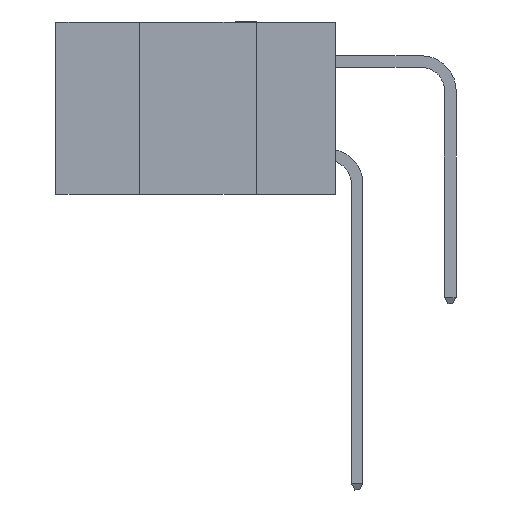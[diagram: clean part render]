
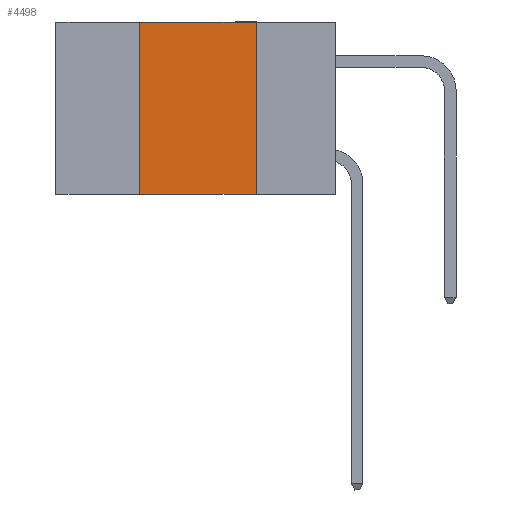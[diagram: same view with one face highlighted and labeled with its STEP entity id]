
A CAD part, left-side view. The second image highlights one B-rep face of the part: STEP entity #4498.
In plain terms, the highlighted planar face has unit normal (-1, 0, 0).
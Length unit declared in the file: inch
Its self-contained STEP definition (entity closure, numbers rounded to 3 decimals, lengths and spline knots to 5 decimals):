
#15 = VECTOR ( 'NONE', #17044, 39.37008 ) ;
#865 = FACE_OUTER_BOUND ( 'NONE', #1380, .T. ) ;
#1380 = EDGE_LOOP ( 'NONE', ( #13947, #5022, #17632, #9290 ) ) ;
#1497 = VECTOR ( 'NONE', #4788, 39.37008 ) ;
#2486 = CARTESIAN_POINT ( 'NONE',  ( 0., 0.42, -0.37 ) ) ;
#2510 = CARTESIAN_POINT ( 'NONE',  ( 0., 0.42, 0. ) ) ;
#3228 = CARTESIAN_POINT ( 'NONE',  ( 0., 0.6, -0.37 ) ) ;
#3567 = EDGE_CURVE ( 'NONE', #5511, #6806, #6130, .T. ) ;
#4498 = ADVANCED_FACE ( 'NONE', ( #865 ), #13098, .F. ) ;
#4788 = DIRECTION ( 'NONE',  ( 0., -1., 0. ) ) ;
#5022 = ORIENTED_EDGE ( 'NONE', *, *, #3567, .F. ) ;
#5511 = VERTEX_POINT ( 'NONE', #2510 ) ;
#6021 = CARTESIAN_POINT ( 'NONE',  ( 0., 0.6, 0. ) ) ;
#6130 = LINE ( 'NONE', #6021, #9954 ) ;
#6806 = VERTEX_POINT ( 'NONE', #15400 ) ;
#8310 = EDGE_CURVE ( 'NONE', #6806, #14572, #15387, .T. ) ;
#8398 = LINE ( 'NONE', #16197, #11627 ) ;
#8873 = AXIS2_PLACEMENT_3D ( 'NONE', #12870, #13113, #12237 ) ;
#9290 = ORIENTED_EDGE ( 'NONE', *, *, #15578, .T. ) ;
#9471 = LINE ( 'NONE', #3228, #1497 ) ;
#9954 = VECTOR ( 'NONE', #17787, 39.37008 ) ;
#11627 = VECTOR ( 'NONE', #12243, 39.37008 ) ;
#12237 = DIRECTION ( 'NONE',  ( 0., 0., -1. ) ) ;
#12243 = DIRECTION ( 'NONE',  ( 0., 0., 1. ) ) ;
#12870 = CARTESIAN_POINT ( 'NONE',  ( 0., 0.6, 0. ) ) ;
#12961 = CARTESIAN_POINT ( 'NONE',  ( 0., 0.17, 0. ) ) ;
#13098 = PLANE ( 'NONE',  #8873 ) ;
#13113 = DIRECTION ( 'NONE',  ( 1., 0., 0. ) ) ;
#13947 = ORIENTED_EDGE ( 'NONE', *, *, #8310, .F. ) ;
#14572 = VERTEX_POINT ( 'NONE', #14808 ) ;
#14808 = CARTESIAN_POINT ( 'NONE',  ( 0., 0.17, -0.37 ) ) ;
#15387 = LINE ( 'NONE', #12961, #15 ) ;
#15400 = CARTESIAN_POINT ( 'NONE',  ( 0., 0.17, 0. ) ) ;
#15578 = EDGE_CURVE ( 'NONE', #17324, #14572, #9471, .T. ) ;
#16197 = CARTESIAN_POINT ( 'NONE',  ( 0., 0.42, 0. ) ) ;
#17044 = DIRECTION ( 'NONE',  ( 0., 0., -1. ) ) ;
#17324 = VERTEX_POINT ( 'NONE', #2486 ) ;
#17632 = ORIENTED_EDGE ( 'NONE', *, *, #18324, .F. ) ;
#17787 = DIRECTION ( 'NONE',  ( 0., -1., 0. ) ) ;
#18324 = EDGE_CURVE ( 'NONE', #17324, #5511, #8398, .T. ) ;
